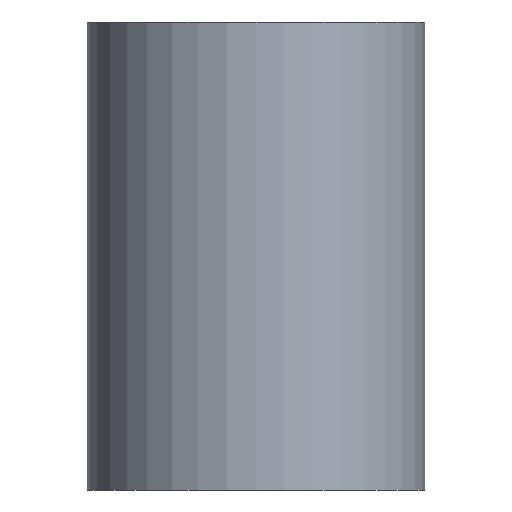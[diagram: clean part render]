
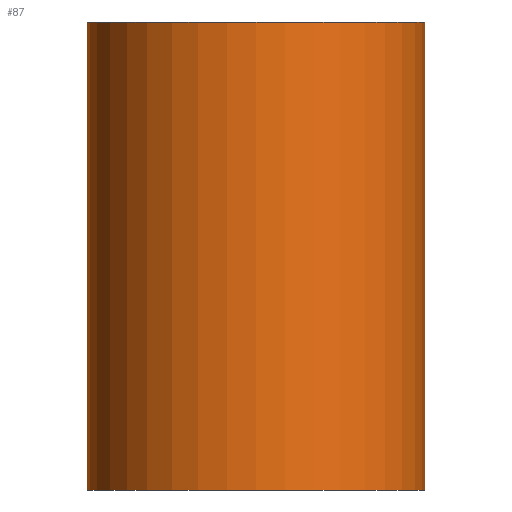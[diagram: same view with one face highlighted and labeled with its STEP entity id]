
A CAD part, front view. The second image highlights one B-rep face of the part: STEP entity #87.
In plain terms, the highlighted cylindrical face has radius 2.381 mm (diameter 4.763 mm), a partial arc.
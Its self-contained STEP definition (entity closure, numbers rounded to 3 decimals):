
#2 = VERTEX_POINT ( 'NONE', #232 ) ;
#5 = LINE ( 'NONE', #206, #190 ) ;
#9 = EDGE_LOOP ( 'NONE', ( #89, #191, #75, #215 ) ) ;
#10 = VERTEX_POINT ( 'NONE', #233 ) ;
#24 = AXIS2_PLACEMENT_3D ( 'NONE', #183, #187, #196 ) ;
#28 = AXIS2_PLACEMENT_3D ( 'NONE', #174, #160, #167 ) ;
#40 = AXIS2_PLACEMENT_3D ( 'NONE', #200, #195, #193 ) ;
#57 = FACE_OUTER_BOUND ( 'NONE', #9, .T. ) ;
#73 = EDGE_CURVE ( 'NONE', #204, #2, #95, .T. ) ;
#75 = ORIENTED_EDGE ( 'NONE', *, *, #80, .T. ) ;
#80 = EDGE_CURVE ( 'NONE', #133, #10, #5, .T. ) ;
#83 = EDGE_CURVE ( 'NONE', #133, #204, #188, .T. ) ;
#87 = ADVANCED_FACE ( 'NONE', ( #57 ), #130, .T. ) ;
#89 = ORIENTED_EDGE ( 'NONE', *, *, #73, .F. ) ;
#95 = LINE ( 'NONE', #247, #98 ) ;
#97 = EDGE_CURVE ( 'NONE', #10, #2, #109, .T. ) ;
#98 = VECTOR ( 'NONE', #239, 1000. ) ;
#109 = CIRCLE ( 'NONE', #28, 2.381 ) ;
#130 = CYLINDRICAL_SURFACE ( 'NONE', #24, 2.381 ) ;
#133 = VERTEX_POINT ( 'NONE', #156 ) ;
#145 = CARTESIAN_POINT ( 'NONE',  ( 2.381, 0., 6.6 ) ) ;
#156 = CARTESIAN_POINT ( 'NONE',  ( -2.381, 0., 6.6 ) ) ;
#160 = DIRECTION ( 'NONE',  ( 0., 0., 1. ) ) ;
#167 = DIRECTION ( 'NONE',  ( 1., 0., 0. ) ) ;
#174 = CARTESIAN_POINT ( 'NONE',  ( 0., 0., 0. ) ) ;
#183 = CARTESIAN_POINT ( 'NONE',  ( 0., 0., 6.6 ) ) ;
#187 = DIRECTION ( 'NONE',  ( 0., 0., -1. ) ) ;
#188 = CIRCLE ( 'NONE', #40, 2.381 ) ;
#190 = VECTOR ( 'NONE', #203, 1000. ) ;
#191 = ORIENTED_EDGE ( 'NONE', *, *, #83, .F. ) ;
#193 = DIRECTION ( 'NONE',  ( 1., 0., 0. ) ) ;
#195 = DIRECTION ( 'NONE',  ( 0., 0., 1. ) ) ;
#196 = DIRECTION ( 'NONE',  ( -1., 0., 0. ) ) ;
#200 = CARTESIAN_POINT ( 'NONE',  ( 0., 0., 6.6 ) ) ;
#203 = DIRECTION ( 'NONE',  ( 0., 0., -1. ) ) ;
#204 = VERTEX_POINT ( 'NONE', #145 ) ;
#206 = CARTESIAN_POINT ( 'NONE',  ( -2.381, 0., 6.6 ) ) ;
#215 = ORIENTED_EDGE ( 'NONE', *, *, #97, .T. ) ;
#232 = CARTESIAN_POINT ( 'NONE',  ( 2.381, 0., 0. ) ) ;
#233 = CARTESIAN_POINT ( 'NONE',  ( -2.381, 0., 0. ) ) ;
#239 = DIRECTION ( 'NONE',  ( 0., 0., -1. ) ) ;
#247 = CARTESIAN_POINT ( 'NONE',  ( 2.381, 0., 6.6 ) ) ;
